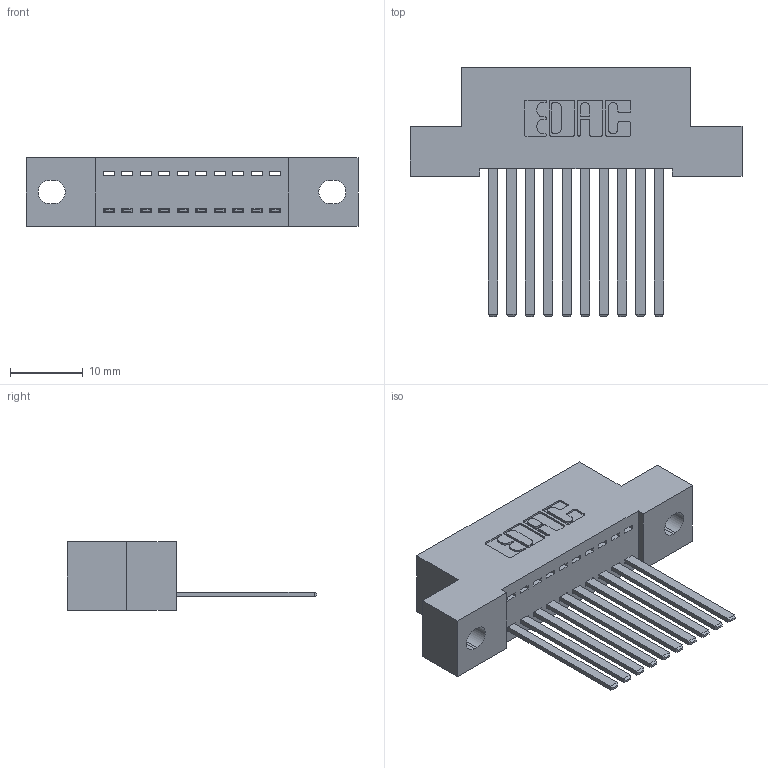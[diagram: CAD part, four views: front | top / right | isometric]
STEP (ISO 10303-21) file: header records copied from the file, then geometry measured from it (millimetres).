
FILE_DESCRIPTION (( 'STEP AP203' ), '1' );
FILE_NAME ('342-010-544-102.STEP', '2019-10-01T14:08:33', ( '' ), ( '' ), 'SwSTEP 2.0', 'SolidWorks 2016', '' );
FILE_SCHEMA (( 'CONFIG_CONTROL_DESIGN' ));
Length unit declared in the file: inch
Products named in the file (3): 342 Part_.128 Slot; 345-292-001_345-293-144; 342-010-544-102
Assembly tree (11 placements, depth 2):
  342-010-544-102
    342 Part_.128 Slot
    345-292-001_345-293-144  x10
Bounding box: 45.72 x 34.3 x 9.4 mm (x, y, z)
Volume: 3954.5 mm3; surface area: 5298.8 mm2
Topology: 11 solids, 11 shells, 634 faces, 1891 edges, 1246 vertices
Faces by surface type: plane 450, cylinder 184
Entity records: 10071 total; most frequent: CARTESIAN_POINT 1748, ORIENTED_EDGE 1694, DIRECTION 1535, EDGE_CURVE 847, VECTOR 723, LINE 723, VERTEX_POINT 562, AXIS2_PLACEMENT_3D 406
